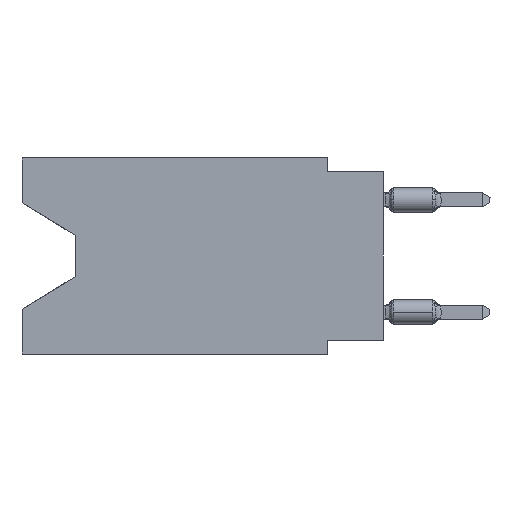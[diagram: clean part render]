
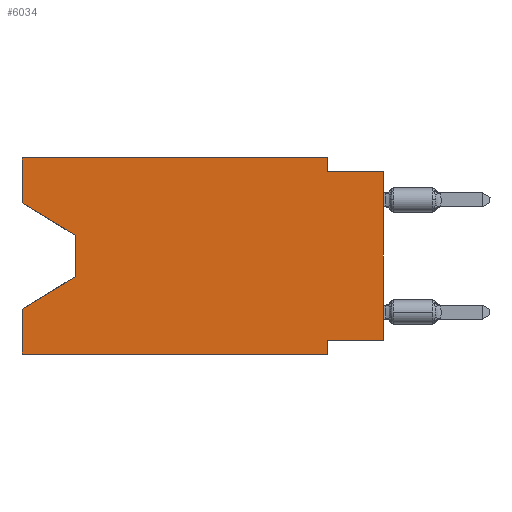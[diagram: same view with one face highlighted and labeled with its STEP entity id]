
A CAD part, left-side view. The second image highlights one B-rep face of the part: STEP entity #6034.
In plain terms, the highlighted planar face has unit normal (-1, 0, 0).
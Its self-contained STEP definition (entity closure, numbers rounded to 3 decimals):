
#94 = DIRECTION ( 'NONE',  ( 0., 0.855, -0.519 ) ) ;
#1176 = CARTESIAN_POINT ( 'NONE',  ( 0., 13.97, -3.505 ) ) ;
#1271 = ORIENTED_EDGE ( 'NONE', *, *, #15047, .F. ) ;
#1626 = EDGE_CURVE ( 'NONE', #24350, #16847, #4534, .T. ) ;
#2312 = ORIENTED_EDGE ( 'NONE', *, *, #1626, .F. ) ;
#2579 = CARTESIAN_POINT ( 'NONE',  ( 0., 2.54, 0. ) ) ;
#3883 = VECTOR ( 'NONE', #50710, 1000. ) ;
#4534 = LINE ( 'NONE', #29961, #32321 ) ;
#4713 = VERTEX_POINT ( 'NONE', #45226 ) ;
#5412 = EDGE_CURVE ( 'NONE', #18211, #49647, #30700, .T. ) ;
#6034 = ADVANCED_FACE ( 'NONE', ( #30003 ), #10062, .F. ) ;
#8194 = CARTESIAN_POINT ( 'NONE',  ( 0., 13.97, -5.385 ) ) ;
#9148 = EDGE_CURVE ( 'NONE', #24350, #34129, #52499, .T. ) ;
#9189 = CARTESIAN_POINT ( 'NONE',  ( 0., 2.54, -0.635 ) ) ;
#9469 = CARTESIAN_POINT ( 'NONE',  ( 0., 2.54, -8.89 ) ) ;
#10062 = PLANE ( 'NONE',  #36303 ) ;
#10745 = LINE ( 'NONE', #11011, #15891 ) ;
#10915 = CARTESIAN_POINT ( 'NONE',  ( 0., 16.383, 0. ) ) ;
#10921 = ORIENTED_EDGE ( 'NONE', *, *, #31832, .F. ) ;
#11011 = CARTESIAN_POINT ( 'NONE',  ( 0., 0., 0. ) ) ;
#11012 = VECTOR ( 'NONE', #46965, 1000. ) ;
#11144 = EDGE_CURVE ( 'NONE', #34129, #31872, #42924, .T. ) ;
#12170 = LINE ( 'NONE', #41518, #28526 ) ;
#12479 = VERTEX_POINT ( 'NONE', #53937 ) ;
#12730 = DIRECTION ( 'NONE',  ( 0., -1., 0. ) ) ;
#13109 = EDGE_CURVE ( 'NONE', #35630, #37992, #49277, .T. ) ;
#13692 = DIRECTION ( 'NONE',  ( 0., 1., 0. ) ) ;
#14579 = ORIENTED_EDGE ( 'NONE', *, *, #13109, .F. ) ;
#14796 = LINE ( 'NONE', #18710, #19778 ) ;
#15047 = EDGE_CURVE ( 'NONE', #12479, #25941, #21091, .T. ) ;
#15093 = CARTESIAN_POINT ( 'NONE',  ( 0., 16.383, -2.038 ) ) ;
#15205 = VECTOR ( 'NONE', #30068, 1000. ) ;
#15891 = VECTOR ( 'NONE', #40918, 1000. ) ;
#16670 = CARTESIAN_POINT ( 'NONE',  ( 0., 13.97, -3.505 ) ) ;
#16847 = VERTEX_POINT ( 'NONE', #10915 ) ;
#17898 = CARTESIAN_POINT ( 'NONE',  ( 0., 13.97, -5.385 ) ) ;
#18211 = VERTEX_POINT ( 'NONE', #43530 ) ;
#18678 = EDGE_LOOP ( 'NONE', ( #47958, #19884, #31039, #1271, #38172, #33026, #30721, #38497, #26767, #14579, #10921, #2312 ) ) ;
#18710 = CARTESIAN_POINT ( 'NONE',  ( 0., 16.383, 0. ) ) ;
#19001 = VECTOR ( 'NONE', #13692, 1000. ) ;
#19778 = VECTOR ( 'NONE', #44137, 1000. ) ;
#19884 = ORIENTED_EDGE ( 'NONE', *, *, #11144, .T. ) ;
#20088 = CARTESIAN_POINT ( 'NONE',  ( 0., 2.54, -8.89 ) ) ;
#21091 = LINE ( 'NONE', #54359, #3883 ) ;
#22130 = EDGE_CURVE ( 'NONE', #37992, #4713, #12170, .T. ) ;
#22370 = CARTESIAN_POINT ( 'NONE',  ( 0., 0., -8.255 ) ) ;
#24350 = VERTEX_POINT ( 'NONE', #15093 ) ;
#25455 = LINE ( 'NONE', #22370, #19001 ) ;
#25788 = EDGE_CURVE ( 'NONE', #46835, #4713, #10745, .T. ) ;
#25941 = VERTEX_POINT ( 'NONE', #52334 ) ;
#26532 = DIRECTION ( 'NONE',  ( 0., 0., -1. ) ) ;
#26767 = ORIENTED_EDGE ( 'NONE', *, *, #22130, .F. ) ;
#28526 = VECTOR ( 'NONE', #12730, 1000. ) ;
#28818 = LINE ( 'NONE', #50067, #11012 ) ;
#29905 = CARTESIAN_POINT ( 'NONE',  ( 0., 2.54, 0. ) ) ;
#29961 = CARTESIAN_POINT ( 'NONE',  ( 0., 16.383, 0. ) ) ;
#30003 = FACE_OUTER_BOUND ( 'NONE', #18678, .T. ) ;
#30068 = DIRECTION ( 'NONE',  ( 0., 0., -1. ) ) ;
#30700 = LINE ( 'NONE', #9469, #41576 ) ;
#30721 = ORIENTED_EDGE ( 'NONE', *, *, #35639, .F. ) ;
#31039 = ORIENTED_EDGE ( 'NONE', *, *, #36399, .T. ) ;
#31832 = EDGE_CURVE ( 'NONE', #16847, #35630, #14796, .T. ) ;
#31872 = VERTEX_POINT ( 'NONE', #17898 ) ;
#32321 = VECTOR ( 'NONE', #42536, 1000. ) ;
#33026 = ORIENTED_EDGE ( 'NONE', *, *, #5412, .F. ) ;
#34129 = VERTEX_POINT ( 'NONE', #1176 ) ;
#34750 = CARTESIAN_POINT ( 'NONE',  ( 0., 0., -8.255 ) ) ;
#35630 = VERTEX_POINT ( 'NONE', #29905 ) ;
#35639 = EDGE_CURVE ( 'NONE', #46835, #18211, #25455, .T. ) ;
#36303 = AXIS2_PLACEMENT_3D ( 'NONE', #48365, #47059, #48635 ) ;
#36399 = EDGE_CURVE ( 'NONE', #31872, #25941, #55172, .T. ) ;
#37992 = VERTEX_POINT ( 'NONE', #9189 ) ;
#38172 = ORIENTED_EDGE ( 'NONE', *, *, #54982, .T. ) ;
#38497 = ORIENTED_EDGE ( 'NONE', *, *, #25788, .T. ) ;
#39115 = VECTOR ( 'NONE', #42993, 1000. ) ;
#39356 = CARTESIAN_POINT ( 'NONE',  ( 0., 16.383, -2.038 ) ) ;
#40587 = DIRECTION ( 'NONE',  ( 0., 0., -1. ) ) ;
#40918 = DIRECTION ( 'NONE',  ( 0., 0., 1. ) ) ;
#41518 = CARTESIAN_POINT ( 'NONE',  ( 0., 0., -0.635 ) ) ;
#41576 = VECTOR ( 'NONE', #26532, 1000. ) ;
#42536 = DIRECTION ( 'NONE',  ( 0., 0., 1. ) ) ;
#42924 = LINE ( 'NONE', #16670, #15205 ) ;
#42993 = DIRECTION ( 'NONE',  ( 0., -0.855, -0.519 ) ) ;
#43530 = CARTESIAN_POINT ( 'NONE',  ( 0., 2.54, -8.255 ) ) ;
#44137 = DIRECTION ( 'NONE',  ( 0., -1., 0. ) ) ;
#45226 = CARTESIAN_POINT ( 'NONE',  ( 0., 0., -0.635 ) ) ;
#46835 = VERTEX_POINT ( 'NONE', #34750 ) ;
#46965 = DIRECTION ( 'NONE',  ( 0., -1., 0. ) ) ;
#47059 = DIRECTION ( 'NONE',  ( 1., 0., 0. ) ) ;
#47958 = ORIENTED_EDGE ( 'NONE', *, *, #9148, .T. ) ;
#48365 = CARTESIAN_POINT ( 'NONE',  ( 0., 16.383, 0. ) ) ;
#48635 = DIRECTION ( 'NONE',  ( 0., 0., -1. ) ) ;
#49277 = LINE ( 'NONE', #2579, #54024 ) ;
#49647 = VERTEX_POINT ( 'NONE', #20088 ) ;
#50067 = CARTESIAN_POINT ( 'NONE',  ( 0., 16.383, -8.89 ) ) ;
#50710 = DIRECTION ( 'NONE',  ( 0., 0., 1. ) ) ;
#52334 = CARTESIAN_POINT ( 'NONE',  ( 0., 16.383, -6.852 ) ) ;
#52499 = LINE ( 'NONE', #39356, #39115 ) ;
#53005 = VECTOR ( 'NONE', #94, 1000. ) ;
#53937 = CARTESIAN_POINT ( 'NONE',  ( 0., 16.383, -8.89 ) ) ;
#54024 = VECTOR ( 'NONE', #40587, 1000. ) ;
#54359 = CARTESIAN_POINT ( 'NONE',  ( 0., 16.383, 0. ) ) ;
#54982 = EDGE_CURVE ( 'NONE', #12479, #49647, #28818, .T. ) ;
#55172 = LINE ( 'NONE', #8194, #53005 ) ;
